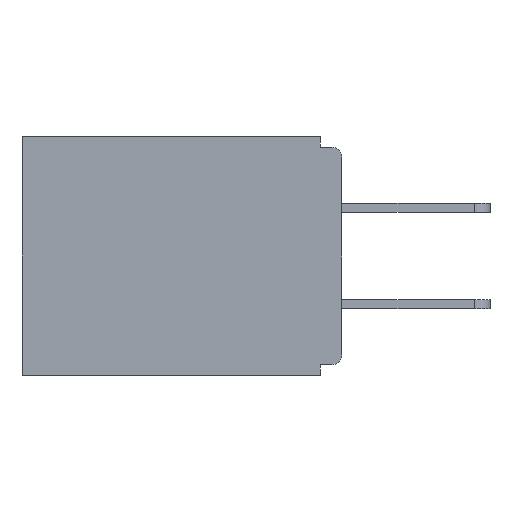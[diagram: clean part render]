
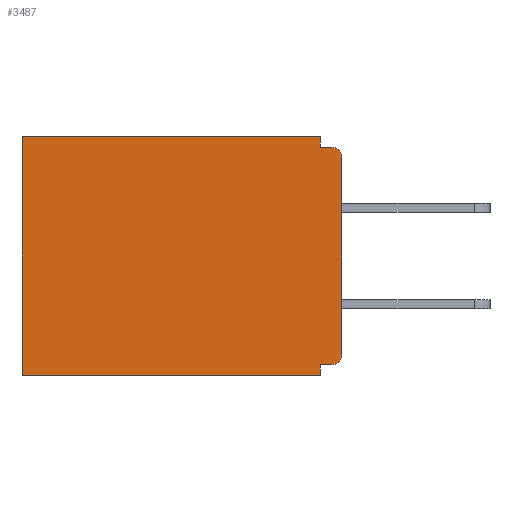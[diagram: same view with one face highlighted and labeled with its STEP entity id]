
A CAD part, left-side view. The second image highlights one B-rep face of the part: STEP entity #3487.
In plain terms, the highlighted planar face has unit normal (-1, 0, 0).
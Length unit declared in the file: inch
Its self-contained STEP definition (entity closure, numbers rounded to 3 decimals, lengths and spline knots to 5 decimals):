
#345 = CARTESIAN_POINT ( 'NONE',  ( 0.298, 0.46, 0. ) ) ;
#612 = CARTESIAN_POINT ( 'NONE',  ( 0.298, 0., -0.03 ) ) ;
#1085 = VERTEX_POINT ( 'NONE', #9936 ) ;
#1394 = ORIENTED_EDGE ( 'NONE', *, *, #6871, .F. ) ;
#2173 = ORIENTED_EDGE ( 'NONE', *, *, #4725, .F. ) ;
#2215 = LINE ( 'NONE', #14929, #13483 ) ;
#2575 = DIRECTION ( 'NONE',  ( 0., 1., 0. ) ) ;
#2597 = CARTESIAN_POINT ( 'NONE',  ( 0.298, 0., 0. ) ) ;
#2707 = CIRCLE ( 'NONE', #17448, 0.015 ) ;
#3299 = ORIENTED_EDGE ( 'NONE', *, *, #7782, .F. ) ;
#3444 = DIRECTION ( 'NONE',  ( 0., 1., 0. ) ) ;
#3487 = ADVANCED_FACE ( 'NONE', ( #4557 ), #6838, .F. ) ;
#3553 = VECTOR ( 'NONE', #2575, 39.37008 ) ;
#3600 = EDGE_CURVE ( 'NONE', #1085, #10850, #6860, .T. ) ;
#3663 = EDGE_CURVE ( 'NONE', #1085, #18275, #2707, .T. ) ;
#3694 = VERTEX_POINT ( 'NONE', #11856 ) ;
#3871 = ORIENTED_EDGE ( 'NONE', *, *, #6423, .F. ) ;
#3986 = DIRECTION ( 'NONE',  ( -1., 0., 0. ) ) ;
#4510 = DIRECTION ( 'NONE',  ( -1., 0., 0. ) ) ;
#4557 = FACE_OUTER_BOUND ( 'NONE', #13264, .T. ) ;
#4725 = EDGE_CURVE ( 'NONE', #5188, #11529, #2215, .T. ) ;
#4763 = CARTESIAN_POINT ( 'NONE',  ( 0.298, 0.031, 0. ) ) ;
#5161 = CARTESIAN_POINT ( 'NONE',  ( 0.298, 0., -0.313 ) ) ;
#5188 = VERTEX_POINT ( 'NONE', #4763 ) ;
#5400 = VECTOR ( 'NONE', #7755, 39.37008 ) ;
#5530 = DIRECTION ( 'NONE',  ( 0., 0., -1. ) ) ;
#6311 = ORIENTED_EDGE ( 'NONE', *, *, #3600, .F. ) ;
#6423 = EDGE_CURVE ( 'NONE', #3694, #13912, #12552, .T. ) ;
#6491 = LINE ( 'NONE', #15226, #9923 ) ;
#6759 = CARTESIAN_POINT ( 'NONE',  ( 0.298, 0.46, -0.343 ) ) ;
#6838 = PLANE ( 'NONE',  #11995 ) ;
#6860 = LINE ( 'NONE', #17487, #17036 ) ;
#6871 = EDGE_CURVE ( 'NONE', #10850, #3694, #15336, .T. ) ;
#7171 = CIRCLE ( 'NONE', #16383, 0.015 ) ;
#7248 = DIRECTION ( 'NONE',  ( 1., 0., 0. ) ) ;
#7417 = VECTOR ( 'NONE', #14658, 39.37008 ) ;
#7638 = EDGE_CURVE ( 'NONE', #5188, #15870, #6491, .T. ) ;
#7755 = DIRECTION ( 'NONE',  ( 0., 0., -1. ) ) ;
#7782 = EDGE_CURVE ( 'NONE', #11529, #15713, #8525, .T. ) ;
#8525 = LINE ( 'NONE', #9990, #18930 ) ;
#8678 = DIRECTION ( 'NONE',  ( 0., 0., -1. ) ) ;
#9914 = DIRECTION ( 'NONE',  ( 0., 1., 0. ) ) ;
#9923 = VECTOR ( 'NONE', #3444, 39.37008 ) ;
#9936 = CARTESIAN_POINT ( 'NONE',  ( 0.298, 0.015, -0.328 ) ) ;
#9990 = CARTESIAN_POINT ( 'NONE',  ( 0.298, 0., -0.015 ) ) ;
#10224 = LINE ( 'NONE', #12298, #5400 ) ;
#10850 = VERTEX_POINT ( 'NONE', #15255 ) ;
#11168 = DIRECTION ( 'NONE',  ( 0., -1., 0. ) ) ;
#11529 = VERTEX_POINT ( 'NONE', #15354 ) ;
#11726 = DIRECTION ( 'NONE',  ( 0., 0., -1. ) ) ;
#11774 = CARTESIAN_POINT ( 'NONE',  ( 0.298, 0.015, -0.015 ) ) ;
#11856 = CARTESIAN_POINT ( 'NONE',  ( 0.298, 0.031, -0.343 ) ) ;
#11995 = AXIS2_PLACEMENT_3D ( 'NONE', #2597, #7248, #8678 ) ;
#12298 = CARTESIAN_POINT ( 'NONE',  ( 0.298, 0., 0. ) ) ;
#12552 = LINE ( 'NONE', #12996, #3553 ) ;
#12881 = EDGE_CURVE ( 'NONE', #14233, #18275, #10224, .T. ) ;
#12933 = CARTESIAN_POINT ( 'NONE',  ( 0.298, 0.015, -0.03 ) ) ;
#12996 = CARTESIAN_POINT ( 'NONE',  ( 0.298, 0., -0.343 ) ) ;
#13229 = LINE ( 'NONE', #16087, #18775 ) ;
#13264 = EDGE_LOOP ( 'NONE', ( #15568, #3299, #2173, #15269, #16558, #3871, #1394, #6311, #14454, #17213 ) ) ;
#13483 = VECTOR ( 'NONE', #15052, 39.37008 ) ;
#13912 = VERTEX_POINT ( 'NONE', #6759 ) ;
#14233 = VERTEX_POINT ( 'NONE', #612 ) ;
#14322 = CARTESIAN_POINT ( 'NONE',  ( 0.298, 0.031, -0.343 ) ) ;
#14454 = ORIENTED_EDGE ( 'NONE', *, *, #3663, .T. ) ;
#14658 = DIRECTION ( 'NONE',  ( 0., 0., -1. ) ) ;
#14929 = CARTESIAN_POINT ( 'NONE',  ( 0.298, 0.031, -0.343 ) ) ;
#15052 = DIRECTION ( 'NONE',  ( 0., 0., -1. ) ) ;
#15122 = EDGE_CURVE ( 'NONE', #15870, #13912, #13229, .T. ) ;
#15226 = CARTESIAN_POINT ( 'NONE',  ( 0.298, 0., 0. ) ) ;
#15255 = CARTESIAN_POINT ( 'NONE',  ( 0.298, 0.031, -0.328 ) ) ;
#15269 = ORIENTED_EDGE ( 'NONE', *, *, #7638, .T. ) ;
#15336 = LINE ( 'NONE', #14322, #7417 ) ;
#15354 = CARTESIAN_POINT ( 'NONE',  ( 0.298, 0.031, -0.015 ) ) ;
#15568 = ORIENTED_EDGE ( 'NONE', *, *, #15673, .T. ) ;
#15673 = EDGE_CURVE ( 'NONE', #14233, #15713, #7171, .T. ) ;
#15713 = VERTEX_POINT ( 'NONE', #11774 ) ;
#15870 = VERTEX_POINT ( 'NONE', #345 ) ;
#16087 = CARTESIAN_POINT ( 'NONE',  ( 0.298, 0.46, 0. ) ) ;
#16209 = DIRECTION ( 'NONE',  ( 0., 0., -1. ) ) ;
#16383 = AXIS2_PLACEMENT_3D ( 'NONE', #12933, #3986, #5530 ) ;
#16558 = ORIENTED_EDGE ( 'NONE', *, *, #15122, .T. ) ;
#17036 = VECTOR ( 'NONE', #9914, 39.37008 ) ;
#17213 = ORIENTED_EDGE ( 'NONE', *, *, #12881, .F. ) ;
#17448 = AXIS2_PLACEMENT_3D ( 'NONE', #17945, #4510, #16209 ) ;
#17487 = CARTESIAN_POINT ( 'NONE',  ( 0.298, 0., -0.328 ) ) ;
#17945 = CARTESIAN_POINT ( 'NONE',  ( 0.298, 0.015, -0.313 ) ) ;
#18275 = VERTEX_POINT ( 'NONE', #5161 ) ;
#18775 = VECTOR ( 'NONE', #11726, 39.37008 ) ;
#18930 = VECTOR ( 'NONE', #11168, 39.37008 ) ;
